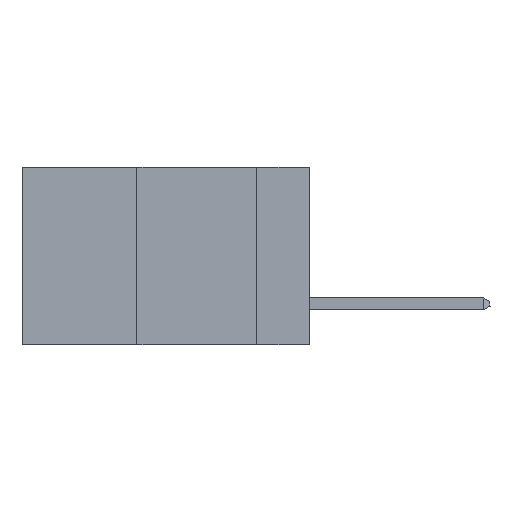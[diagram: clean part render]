
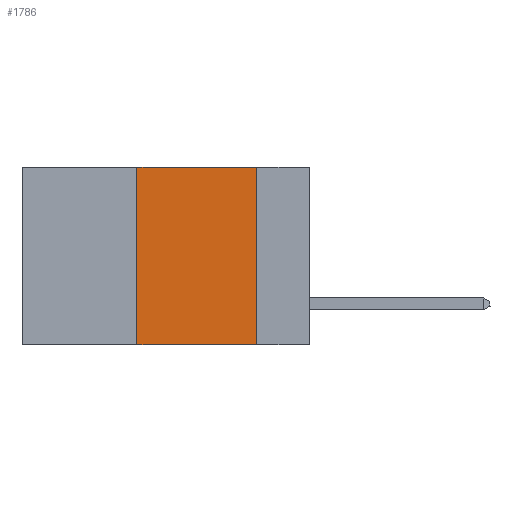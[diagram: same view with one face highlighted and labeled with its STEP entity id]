
A CAD part, left-side view. The second image highlights one B-rep face of the part: STEP entity #1786.
In plain terms, the highlighted planar face has unit normal (-1, 0, 0).
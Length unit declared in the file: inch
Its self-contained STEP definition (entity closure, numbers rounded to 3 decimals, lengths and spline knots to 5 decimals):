
#1610 = VECTOR ( 'NONE', #49807, 39.37008 ) ;
#1786 = ADVANCED_FACE ( 'NONE', ( #30968 ), #31118, .F. ) ;
#3126 = DIRECTION ( 'NONE',  ( 0., 0., 1. ) ) ;
#5254 = ORIENTED_EDGE ( 'NONE', *, *, #9803, .F. ) ;
#5915 = LINE ( 'NONE', #45694, #1610 ) ;
#6326 = DIRECTION ( 'NONE',  ( 0., 0., -1. ) ) ;
#6710 = CARTESIAN_POINT ( 'NONE',  ( 0., 0.6, -0.37 ) ) ;
#9193 = LINE ( 'NONE', #6710, #43816 ) ;
#9803 = EDGE_CURVE ( 'NONE', #20476, #32994, #5915, .T. ) ;
#12765 = EDGE_CURVE ( 'NONE', #20250, #32994, #9193, .T. ) ;
#14509 = EDGE_LOOP ( 'NONE', ( #5254, #28800, #38564, #42330 ) ) ;
#15365 = LINE ( 'NONE', #25054, #35983 ) ;
#15490 = CARTESIAN_POINT ( 'NONE',  ( 0., 0.11, -0.37 ) ) ;
#19487 = CARTESIAN_POINT ( 'NONE',  ( 0., 0.11, 0. ) ) ;
#20250 = VERTEX_POINT ( 'NONE', #40440 ) ;
#20476 = VERTEX_POINT ( 'NONE', #19487 ) ;
#21406 = CARTESIAN_POINT ( 'NONE',  ( 0., 0.6, 0. ) ) ;
#22465 = VECTOR ( 'NONE', #3126, 39.37008 ) ;
#25054 = CARTESIAN_POINT ( 'NONE',  ( 0., 0.6, 0. ) ) ;
#26203 = DIRECTION ( 'NONE',  ( 0., -1., 0. ) ) ;
#26386 = CARTESIAN_POINT ( 'NONE',  ( 0., 0.36, 0. ) ) ;
#28800 = ORIENTED_EDGE ( 'NONE', *, *, #41048, .F. ) ;
#30968 = FACE_OUTER_BOUND ( 'NONE', #14509, .T. ) ;
#31118 = PLANE ( 'NONE',  #34753 ) ;
#32766 = LINE ( 'NONE', #26386, #22465 ) ;
#32900 = EDGE_CURVE ( 'NONE', #20250, #49909, #32766, .T. ) ;
#32994 = VERTEX_POINT ( 'NONE', #15490 ) ;
#34753 = AXIS2_PLACEMENT_3D ( 'NONE', #21406, #39753, #6326 ) ;
#35983 = VECTOR ( 'NONE', #48119, 39.37008 ) ;
#38564 = ORIENTED_EDGE ( 'NONE', *, *, #32900, .F. ) ;
#39753 = DIRECTION ( 'NONE',  ( 1., 0., 0. ) ) ;
#40440 = CARTESIAN_POINT ( 'NONE',  ( 0., 0.36, -0.37 ) ) ;
#41048 = EDGE_CURVE ( 'NONE', #49909, #20476, #15365, .T. ) ;
#42330 = ORIENTED_EDGE ( 'NONE', *, *, #12765, .T. ) ;
#43816 = VECTOR ( 'NONE', #26203, 39.37008 ) ;
#45694 = CARTESIAN_POINT ( 'NONE',  ( 0., 0.11, 0. ) ) ;
#46428 = CARTESIAN_POINT ( 'NONE',  ( 0., 0.36, 0. ) ) ;
#48119 = DIRECTION ( 'NONE',  ( 0., -1., 0. ) ) ;
#49807 = DIRECTION ( 'NONE',  ( 0., 0., -1. ) ) ;
#49909 = VERTEX_POINT ( 'NONE', #46428 ) ;
